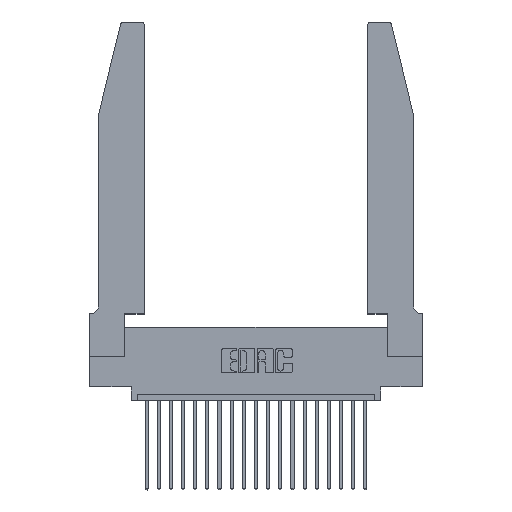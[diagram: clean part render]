
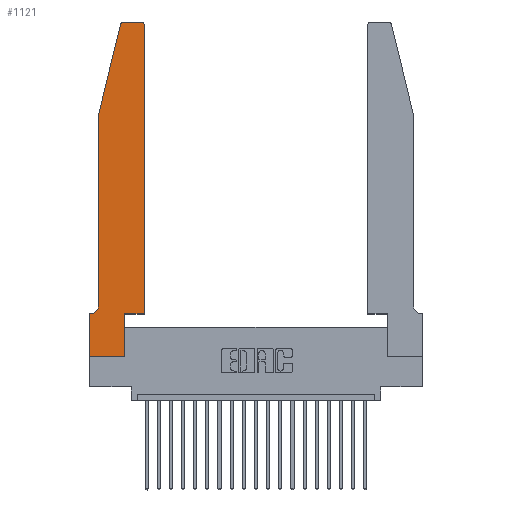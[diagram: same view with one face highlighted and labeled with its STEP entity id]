
A CAD part, top view. The second image highlights one B-rep face of the part: STEP entity #1121.
In plain terms, the highlighted planar face has unit normal (0, 0, 1).
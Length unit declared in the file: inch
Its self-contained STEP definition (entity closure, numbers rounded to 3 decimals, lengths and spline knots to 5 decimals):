
#437 = DIRECTION ( 'NONE',  ( 0., 0., 1. ) ) ;
#921 = VERTEX_POINT ( 'NONE', #8302 ) ;
#1121 = ADVANCED_FACE ( 'NONE', ( #20348 ), #5557, .T. ) ;
#1359 = CARTESIAN_POINT ( 'NONE',  ( 0.4505, 2.72, 0.37 ) ) ;
#1407 = AXIS2_PLACEMENT_3D ( 'NONE', #7786, #9146, #4266 ) ;
#1904 = CARTESIAN_POINT ( 'NONE',  ( 0.0755, 2., 0.37 ) ) ;
#1949 = ORIENTED_EDGE ( 'NONE', *, *, #3034, .T. ) ;
#2134 = CARTESIAN_POINT ( 'NONE',  ( 0.0055, 0.35, 0.37 ) ) ;
#2253 = DIRECTION ( 'NONE',  ( 1., 0., 0. ) ) ;
#2662 = CARTESIAN_POINT ( 'NONE',  ( 0.0755, 0.35, 0.37 ) ) ;
#2784 = CARTESIAN_POINT ( 'NONE',  ( 0.284, 2.75, 0.37 ) ) ;
#3034 = EDGE_CURVE ( 'NONE', #19164, #20713, #13334, .T. ) ;
#3190 = VECTOR ( 'NONE', #19253, 39.37008 ) ;
#3311 = VERTEX_POINT ( 'NONE', #17961 ) ;
#3348 = LINE ( 'NONE', #9022, #6324 ) ;
#3641 = VECTOR ( 'NONE', #19788, 39.37008 ) ;
#3778 = DIRECTION ( 'NONE',  ( 0., 0., -1. ) ) ;
#3890 = DIRECTION ( 'NONE',  ( 1., 0., 0. ) ) ;
#3908 = ORIENTED_EDGE ( 'NONE', *, *, #21550, .T. ) ;
#3951 = ORIENTED_EDGE ( 'NONE', *, *, #15426, .T. ) ;
#4060 = EDGE_CURVE ( 'NONE', #11671, #14535, #6826, .T. ) ;
#4253 = EDGE_CURVE ( 'NONE', #15100, #7881, #15660, .T. ) ;
#4266 = DIRECTION ( 'NONE',  ( 1., 0., 0. ) ) ;
#4307 = DIRECTION ( 'NONE',  ( 0., 1., 0. ) ) ;
#4401 = VECTOR ( 'NONE', #10429, 39.37008 ) ;
#5029 = DIRECTION ( 'NONE',  ( 0., 1., 0. ) ) ;
#5312 = EDGE_CURVE ( 'NONE', #14535, #19164, #11637, .T. ) ;
#5557 = PLANE ( 'NONE',  #16202 ) ;
#5598 = CARTESIAN_POINT ( 'NONE',  ( 0., 0., 0.37 ) ) ;
#6131 = EDGE_LOOP ( 'NONE', ( #15254, #21610, #13721, #8914, #19927, #20237, #3908, #3951, #9501, #10117, #1949, #7830 ) ) ;
#6324 = VECTOR ( 'NONE', #13805, 39.37008 ) ;
#6512 = AXIS2_PLACEMENT_3D ( 'NONE', #17485, #3778, #15757 ) ;
#6547 = LINE ( 'NONE', #18877, #19987 ) ;
#6826 = LINE ( 'NONE', #18254, #10845 ) ;
#7297 = CARTESIAN_POINT ( 'NONE',  ( 0.4505, 0.35, 0.37 ) ) ;
#7510 = CARTESIAN_POINT ( 'NONE',  ( 0., 0.35, 0.37 ) ) ;
#7786 = CARTESIAN_POINT ( 'NONE',  ( 0.4205, 2.72, 0.37 ) ) ;
#7830 = ORIENTED_EDGE ( 'NONE', *, *, #19838, .T. ) ;
#7881 = VERTEX_POINT ( 'NONE', #1904 ) ;
#8048 = CARTESIAN_POINT ( 'NONE',  ( 0.25487, 2.72718, 0.37 ) ) ;
#8072 = CARTESIAN_POINT ( 'NONE',  ( 0.4505, 0.35, 0.37 ) ) ;
#8099 = VERTEX_POINT ( 'NONE', #19310 ) ;
#8302 = CARTESIAN_POINT ( 'NONE',  ( 0., 0., 0.37 ) ) ;
#8583 = CARTESIAN_POINT ( 'NONE',  ( 0.0755, 2., 0.37 ) ) ;
#8914 = ORIENTED_EDGE ( 'NONE', *, *, #21721, .T. ) ;
#9022 = CARTESIAN_POINT ( 'NONE',  ( 0.0755, 2., 0.37 ) ) ;
#9146 = DIRECTION ( 'NONE',  ( 0., 0., 1. ) ) ;
#9482 = VERTEX_POINT ( 'NONE', #2784 ) ;
#9501 = ORIENTED_EDGE ( 'NONE', *, *, #4060, .T. ) ;
#9846 = CIRCLE ( 'NONE', #17500, 0.03 ) ;
#10117 = ORIENTED_EDGE ( 'NONE', *, *, #5312, .T. ) ;
#10429 = DIRECTION ( 'NONE',  ( -0.239, -0.971, 0. ) ) ;
#10595 = LINE ( 'NONE', #16684, #13836 ) ;
#10845 = VECTOR ( 'NONE', #4307, 39.37008 ) ;
#11637 = LINE ( 'NONE', #7297, #20490 ) ;
#11671 = VERTEX_POINT ( 'NONE', #19787 ) ;
#11704 = VECTOR ( 'NONE', #5029, 39.37008 ) ;
#11761 = EDGE_CURVE ( 'NONE', #8099, #9482, #6547, .T. ) ;
#12295 = CARTESIAN_POINT ( 'NONE',  ( 0.2865, 0.35, 0.37 ) ) ;
#12435 = DIRECTION ( 'NONE',  ( 0., 0., 1. ) ) ;
#13240 = CARTESIAN_POINT ( 'NONE',  ( 0.284, 2.72, 0.37 ) ) ;
#13334 = LINE ( 'NONE', #17083, #11704 ) ;
#13554 = LINE ( 'NONE', #2662, #3641 ) ;
#13721 = ORIENTED_EDGE ( 'NONE', *, *, #4253, .T. ) ;
#13758 = VERTEX_POINT ( 'NONE', #15313 ) ;
#13805 = DIRECTION ( 'NONE',  ( 0., -1., 0. ) ) ;
#13836 = VECTOR ( 'NONE', #20395, 39.37008 ) ;
#14535 = VERTEX_POINT ( 'NONE', #12295 ) ;
#15100 = VERTEX_POINT ( 'NONE', #8048 ) ;
#15254 = ORIENTED_EDGE ( 'NONE', *, *, #11761, .T. ) ;
#15313 = CARTESIAN_POINT ( 'NONE',  ( 0., 0.35, 0.37 ) ) ;
#15426 = EDGE_CURVE ( 'NONE', #921, #11671, #20385, .T. ) ;
#15660 = LINE ( 'NONE', #8583, #4401 ) ;
#15757 = DIRECTION ( 'NONE',  ( -1., 0., 0. ) ) ;
#15879 = DIRECTION ( 'NONE',  ( 1., 0., 0. ) ) ;
#16202 = AXIS2_PLACEMENT_3D ( 'NONE', #7510, #437, #15879 ) ;
#16241 = CIRCLE ( 'NONE', #6512, 0.07 ) ;
#16684 = CARTESIAN_POINT ( 'NONE',  ( 0., 0., 0.37 ) ) ;
#16866 = VERTEX_POINT ( 'NONE', #2134 ) ;
#16954 = CIRCLE ( 'NONE', #1407, 0.03 ) ;
#16994 = EDGE_CURVE ( 'NONE', #9482, #15100, #9846, .T. ) ;
#17083 = CARTESIAN_POINT ( 'NONE',  ( 0.4505, 0.35, 0.37 ) ) ;
#17485 = CARTESIAN_POINT ( 'NONE',  ( 0.0055, 0.42, 0.37 ) ) ;
#17500 = AXIS2_PLACEMENT_3D ( 'NONE', #13240, #12435, #3890 ) ;
#17961 = CARTESIAN_POINT ( 'NONE',  ( 0.0755, 0.42, 0.37 ) ) ;
#18254 = CARTESIAN_POINT ( 'NONE',  ( 0.2865, 0.35, 0.37 ) ) ;
#18877 = CARTESIAN_POINT ( 'NONE',  ( 0.2605, 2.75, 0.37 ) ) ;
#19025 = DIRECTION ( 'NONE',  ( -1., 0., 0. ) ) ;
#19164 = VERTEX_POINT ( 'NONE', #8072 ) ;
#19253 = DIRECTION ( 'NONE',  ( 1., 0., 0. ) ) ;
#19310 = CARTESIAN_POINT ( 'NONE',  ( 0.4205, 2.75, 0.37 ) ) ;
#19787 = CARTESIAN_POINT ( 'NONE',  ( 0.2865, 0., 0.37 ) ) ;
#19788 = DIRECTION ( 'NONE',  ( -1., 0., 0. ) ) ;
#19838 = EDGE_CURVE ( 'NONE', #20713, #8099, #16954, .T. ) ;
#19927 = ORIENTED_EDGE ( 'NONE', *, *, #21066, .T. ) ;
#19987 = VECTOR ( 'NONE', #19025, 39.37008 ) ;
#20237 = ORIENTED_EDGE ( 'NONE', *, *, #21508, .T. ) ;
#20348 = FACE_OUTER_BOUND ( 'NONE', #6131, .T. ) ;
#20385 = LINE ( 'NONE', #5598, #3190 ) ;
#20395 = DIRECTION ( 'NONE',  ( 0., -1., 0. ) ) ;
#20490 = VECTOR ( 'NONE', #2253, 39.37008 ) ;
#20713 = VERTEX_POINT ( 'NONE', #1359 ) ;
#21066 = EDGE_CURVE ( 'NONE', #3311, #16866, #16241, .T. ) ;
#21508 = EDGE_CURVE ( 'NONE', #16866, #13758, #13554, .T. ) ;
#21550 = EDGE_CURVE ( 'NONE', #13758, #921, #10595, .T. ) ;
#21610 = ORIENTED_EDGE ( 'NONE', *, *, #16994, .T. ) ;
#21721 = EDGE_CURVE ( 'NONE', #7881, #3311, #3348, .T. ) ;
